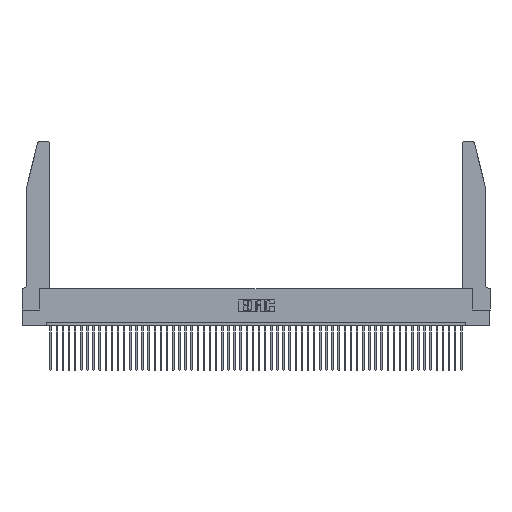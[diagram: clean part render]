
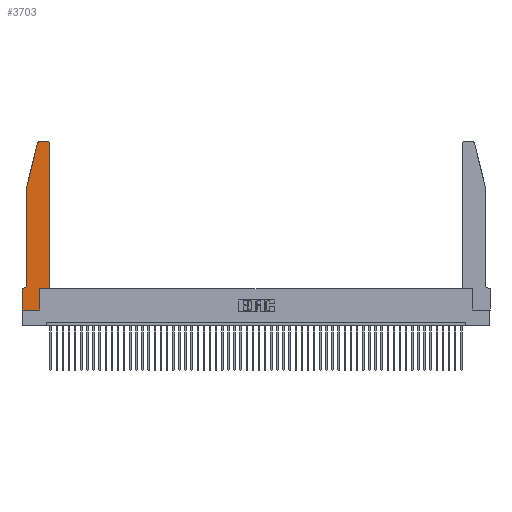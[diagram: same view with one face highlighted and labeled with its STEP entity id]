
A CAD part, top view. The second image highlights one B-rep face of the part: STEP entity #3703.
In plain terms, the highlighted planar face has unit normal (0, 0, 1).
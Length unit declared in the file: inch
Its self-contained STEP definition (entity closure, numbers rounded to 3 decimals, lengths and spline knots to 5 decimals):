
#1024 = VECTOR ( 'NONE', #31061, 39.37008 ) ;
#1250 = AXIS2_PLACEMENT_3D ( 'NONE', #39381, #39189, #27302 ) ;
#2124 = ORIENTED_EDGE ( 'NONE', *, *, #49864, .T. ) ;
#2304 = LINE ( 'NONE', #23210, #24464 ) ;
#2650 = CARTESIAN_POINT ( 'NONE',  ( 0.4505, 2.72, 0.37 ) ) ;
#3423 = VERTEX_POINT ( 'NONE', #46058 ) ;
#3703 = ADVANCED_FACE ( 'NONE', ( #21332 ), #31395, .T. ) ;
#3865 = DIRECTION ( 'NONE',  ( -0.239, -0.971, 0. ) ) ;
#3984 = CARTESIAN_POINT ( 'NONE',  ( 0.0755, 2., 0.37 ) ) ;
#4246 = VERTEX_POINT ( 'NONE', #15774 ) ;
#5774 = VECTOR ( 'NONE', #32986, 39.37008 ) ;
#6481 = CARTESIAN_POINT ( 'NONE',  ( 0.4505, 0.35, 0.37 ) ) ;
#8386 = DIRECTION ( 'NONE',  ( 1., 0., 0. ) ) ;
#9187 = VERTEX_POINT ( 'NONE', #3984 ) ;
#9810 = CARTESIAN_POINT ( 'NONE',  ( 0.2865, 0.35, 0.37 ) ) ;
#9858 = VECTOR ( 'NONE', #29347, 39.37008 ) ;
#10313 = EDGE_CURVE ( 'NONE', #26052, #19664, #30511, .T. ) ;
#10387 = CIRCLE ( 'NONE', #18304, 0.03 ) ;
#10549 = ORIENTED_EDGE ( 'NONE', *, *, #51812, .T. ) ;
#10810 = LINE ( 'NONE', #38361, #41816 ) ;
#12084 = CARTESIAN_POINT ( 'NONE',  ( 0.0055, 0.42, 0.37 ) ) ;
#12170 = VERTEX_POINT ( 'NONE', #2650 ) ;
#12318 = VECTOR ( 'NONE', #24848, 39.37008 ) ;
#13070 = VERTEX_POINT ( 'NONE', #46495 ) ;
#13327 = EDGE_CURVE ( 'NONE', #13070, #17813, #10810, .T. ) ;
#14025 = EDGE_CURVE ( 'NONE', #46125, #22792, #29721, .T. ) ;
#14193 = CARTESIAN_POINT ( 'NONE',  ( 0., 0., 0.37 ) ) ;
#15774 = CARTESIAN_POINT ( 'NONE',  ( 0.4205, 2.75, 0.37 ) ) ;
#16011 = DIRECTION ( 'NONE',  ( 0., 0., 1. ) ) ;
#16151 = VERTEX_POINT ( 'NONE', #26392 ) ;
#16589 = ORIENTED_EDGE ( 'NONE', *, *, #24127, .T. ) ;
#16973 = ORIENTED_EDGE ( 'NONE', *, *, #48444, .T. ) ;
#17688 = AXIS2_PLACEMENT_3D ( 'NONE', #12084, #24004, #23662 ) ;
#17813 = VERTEX_POINT ( 'NONE', #14193 ) ;
#18304 = AXIS2_PLACEMENT_3D ( 'NONE', #43415, #16011, #8386 ) ;
#19072 = VECTOR ( 'NONE', #20483, 39.37008 ) ;
#19664 = VERTEX_POINT ( 'NONE', #22947 ) ;
#20483 = DIRECTION ( 'NONE',  ( 1., 0., 0. ) ) ;
#20638 = ORIENTED_EDGE ( 'NONE', *, *, #25828, .T. ) ;
#21332 = FACE_OUTER_BOUND ( 'NONE', #26700, .T. ) ;
#21742 = EDGE_CURVE ( 'NONE', #17813, #36471, #30052, .T. ) ;
#21788 = CARTESIAN_POINT ( 'NONE',  ( 0., 0., 0.37 ) ) ;
#21887 = LINE ( 'NONE', #41757, #9858 ) ;
#21966 = DIRECTION ( 'NONE',  ( 1., 0., 0. ) ) ;
#22469 = EDGE_CURVE ( 'NONE', #9187, #3423, #31420, .T. ) ;
#22792 = VERTEX_POINT ( 'NONE', #23259 ) ;
#22947 = CARTESIAN_POINT ( 'NONE',  ( 0.4505, 0.35, 0.37 ) ) ;
#23210 = CARTESIAN_POINT ( 'NONE',  ( 0.0755, 2., 0.37 ) ) ;
#23259 = CARTESIAN_POINT ( 'NONE',  ( 0.25487, 2.72718, 0.37 ) ) ;
#23662 = DIRECTION ( 'NONE',  ( -1., 0., 0. ) ) ;
#24004 = DIRECTION ( 'NONE',  ( 0., 0., -1. ) ) ;
#24127 = EDGE_CURVE ( 'NONE', #4246, #46125, #37871, .T. ) ;
#24464 = VECTOR ( 'NONE', #3865, 39.37008 ) ;
#24848 = DIRECTION ( 'NONE',  ( 0., -1., 0. ) ) ;
#25828 = EDGE_CURVE ( 'NONE', #12170, #4246, #10387, .T. ) ;
#26052 = VERTEX_POINT ( 'NONE', #9810 ) ;
#26392 = CARTESIAN_POINT ( 'NONE',  ( 0.0055, 0.35, 0.37 ) ) ;
#26700 = EDGE_LOOP ( 'NONE', ( #16589, #26905, #33661, #38406, #16973, #10549, #38703, #50517, #2124, #38451, #47867, #20638 ) ) ;
#26905 = ORIENTED_EDGE ( 'NONE', *, *, #14025, .T. ) ;
#26951 = CARTESIAN_POINT ( 'NONE',  ( 0.2605, 2.75, 0.37 ) ) ;
#27125 = CARTESIAN_POINT ( 'NONE',  ( 0.4505, 0.35, 0.37 ) ) ;
#27302 = DIRECTION ( 'NONE',  ( 1., 0., 0. ) ) ;
#28764 = CARTESIAN_POINT ( 'NONE',  ( 0.284, 2.75, 0.37 ) ) ;
#29347 = DIRECTION ( 'NONE',  ( -1., 0., 0. ) ) ;
#29721 = CIRCLE ( 'NONE', #1250, 0.03 ) ;
#30052 = LINE ( 'NONE', #21788, #52292 ) ;
#30511 = LINE ( 'NONE', #27125, #19072 ) ;
#31061 = DIRECTION ( 'NONE',  ( -1., 0., 0. ) ) ;
#31395 = PLANE ( 'NONE',  #36084 ) ;
#31420 = LINE ( 'NONE', #45025, #12318 ) ;
#32986 = DIRECTION ( 'NONE',  ( 0., 1., 0. ) ) ;
#33661 = ORIENTED_EDGE ( 'NONE', *, *, #41195, .T. ) ;
#35599 = EDGE_CURVE ( 'NONE', #19664, #12170, #38169, .T. ) ;
#36084 = AXIS2_PLACEMENT_3D ( 'NONE', #39240, #44489, #37032 ) ;
#36471 = VERTEX_POINT ( 'NONE', #47033 ) ;
#37032 = DIRECTION ( 'NONE',  ( 1., 0., 0. ) ) ;
#37826 = CIRCLE ( 'NONE', #17688, 0.07 ) ;
#37871 = LINE ( 'NONE', #26951, #1024 ) ;
#38169 = LINE ( 'NONE', #6481, #5774 ) ;
#38361 = CARTESIAN_POINT ( 'NONE',  ( 0., 0., 0.37 ) ) ;
#38406 = ORIENTED_EDGE ( 'NONE', *, *, #22469, .T. ) ;
#38451 = ORIENTED_EDGE ( 'NONE', *, *, #10313, .T. ) ;
#38703 = ORIENTED_EDGE ( 'NONE', *, *, #13327, .T. ) ;
#39189 = DIRECTION ( 'NONE',  ( 0., 0., 1. ) ) ;
#39240 = CARTESIAN_POINT ( 'NONE',  ( 0., 0.35, 0.37 ) ) ;
#39381 = CARTESIAN_POINT ( 'NONE',  ( 0.284, 2.72, 0.37 ) ) ;
#41195 = EDGE_CURVE ( 'NONE', #22792, #9187, #2304, .T. ) ;
#41757 = CARTESIAN_POINT ( 'NONE',  ( 0.0755, 0.35, 0.37 ) ) ;
#41816 = VECTOR ( 'NONE', #50883, 39.37008 ) ;
#43415 = CARTESIAN_POINT ( 'NONE',  ( 0.4205, 2.72, 0.37 ) ) ;
#44489 = DIRECTION ( 'NONE',  ( 0., 0., 1. ) ) ;
#45025 = CARTESIAN_POINT ( 'NONE',  ( 0.0755, 2., 0.37 ) ) ;
#45552 = CARTESIAN_POINT ( 'NONE',  ( 0.2865, 0.35, 0.37 ) ) ;
#46058 = CARTESIAN_POINT ( 'NONE',  ( 0.0755, 0.42, 0.37 ) ) ;
#46125 = VERTEX_POINT ( 'NONE', #28764 ) ;
#46495 = CARTESIAN_POINT ( 'NONE',  ( 0., 0.35, 0.37 ) ) ;
#46918 = VECTOR ( 'NONE', #50158, 39.37008 ) ;
#47033 = CARTESIAN_POINT ( 'NONE',  ( 0.2865, 0., 0.37 ) ) ;
#47867 = ORIENTED_EDGE ( 'NONE', *, *, #35599, .T. ) ;
#48222 = LINE ( 'NONE', #45552, #46918 ) ;
#48444 = EDGE_CURVE ( 'NONE', #3423, #16151, #37826, .T. ) ;
#49864 = EDGE_CURVE ( 'NONE', #36471, #26052, #48222, .T. ) ;
#50158 = DIRECTION ( 'NONE',  ( 0., 1., 0. ) ) ;
#50517 = ORIENTED_EDGE ( 'NONE', *, *, #21742, .T. ) ;
#50883 = DIRECTION ( 'NONE',  ( 0., -1., 0. ) ) ;
#51812 = EDGE_CURVE ( 'NONE', #16151, #13070, #21887, .T. ) ;
#52292 = VECTOR ( 'NONE', #21966, 39.37008 ) ;
